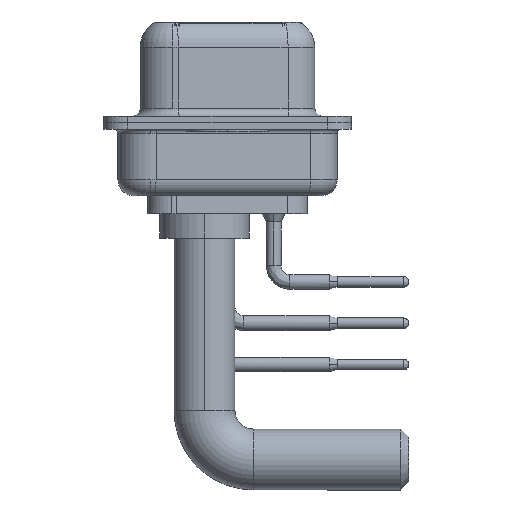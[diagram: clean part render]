
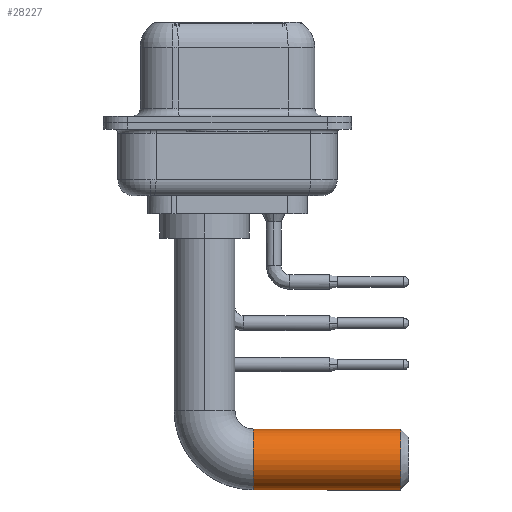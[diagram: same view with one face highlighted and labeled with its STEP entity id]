
A CAD part, left-side view. The second image highlights one B-rep face of the part: STEP entity #28227.
In plain terms, the highlighted cylindrical face has radius 1.875 mm (diameter 3.75 mm), a partial arc.
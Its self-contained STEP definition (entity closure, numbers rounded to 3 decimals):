
#1708 = CIRCLE ( 'NONE', #2202, 1.875 ) ;
#1998 = CARTESIAN_POINT ( 'NONE',  ( 0., -12.07, -15.505 ) ) ;
#2202 = AXIS2_PLACEMENT_3D ( 'NONE', #20396, #3746, #25241 ) ;
#3065 = VERTEX_POINT ( 'NONE', #28035 ) ;
#3083 = EDGE_CURVE ( 'NONE', #12102, #7497, #7373, .T. ) ;
#3746 = DIRECTION ( 'NONE',  ( 0., -1., 0. ) ) ;
#5138 = EDGE_CURVE ( 'NONE', #13464, #3065, #1708, .T. ) ;
#5786 = ORIENTED_EDGE ( 'NONE', *, *, #5138, .T. ) ;
#7333 = VECTOR ( 'NONE', #21240, 1000. ) ;
#7373 = CIRCLE ( 'NONE', #12353, 1.875 ) ;
#7497 = VERTEX_POINT ( 'NONE', #14521 ) ;
#7834 = CYLINDRICAL_SURFACE ( 'NONE', #10019, 1.875 ) ;
#7890 = ORIENTED_EDGE ( 'NONE', *, *, #3083, .T. ) ;
#9256 = LINE ( 'NONE', #28872, #7333 ) ;
#10019 = AXIS2_PLACEMENT_3D ( 'NONE', #29471, #14527, #24177 ) ;
#10800 = EDGE_CURVE ( 'NONE', #3065, #12102, #13676, .T. ) ;
#11531 = CARTESIAN_POINT ( 'NONE',  ( 0., -12.07, -13.63 ) ) ;
#12102 = VERTEX_POINT ( 'NONE', #1998 ) ;
#12353 = AXIS2_PLACEMENT_3D ( 'NONE', #11531, #21015, #30514 ) ;
#13142 = ORIENTED_EDGE ( 'NONE', *, *, #10800, .T. ) ;
#13464 = VERTEX_POINT ( 'NONE', #26597 ) ;
#13676 = LINE ( 'NONE', #21431, #23772 ) ;
#14236 = EDGE_LOOP ( 'NONE', ( #24817, #5786, #13142, #7890 ) ) ;
#14521 = CARTESIAN_POINT ( 'NONE',  ( 0., -12.07, -11.755 ) ) ;
#14527 = DIRECTION ( 'NONE',  ( 0., -1., 0. ) ) ;
#14993 = FACE_OUTER_BOUND ( 'NONE', #14236, .T. ) ;
#16622 = DIRECTION ( 'NONE',  ( 0., -1., 0. ) ) ;
#20396 = CARTESIAN_POINT ( 'NONE',  ( 0., -3., -13.63 ) ) ;
#21015 = DIRECTION ( 'NONE',  ( 0., 1., 0. ) ) ;
#21240 = DIRECTION ( 'NONE',  ( 0., -1., 0. ) ) ;
#21431 = CARTESIAN_POINT ( 'NONE',  ( 0., -3., -15.505 ) ) ;
#22514 = EDGE_CURVE ( 'NONE', #13464, #7497, #9256, .T. ) ;
#23772 = VECTOR ( 'NONE', #16622, 1000. ) ;
#24177 = DIRECTION ( 'NONE',  ( 0., 0., -1. ) ) ;
#24817 = ORIENTED_EDGE ( 'NONE', *, *, #22514, .F. ) ;
#25241 = DIRECTION ( 'NONE',  ( -1., 0., 0. ) ) ;
#26597 = CARTESIAN_POINT ( 'NONE',  ( 0., -3., -11.755 ) ) ;
#28035 = CARTESIAN_POINT ( 'NONE',  ( 0., -3., -15.505 ) ) ;
#28227 = ADVANCED_FACE ( 'NONE', ( #14993 ), #7834, .T. ) ;
#28872 = CARTESIAN_POINT ( 'NONE',  ( 0., -3., -11.755 ) ) ;
#29471 = CARTESIAN_POINT ( 'NONE',  ( 0., -3., -13.63 ) ) ;
#30514 = DIRECTION ( 'NONE',  ( 0., 0., -1. ) ) ;
